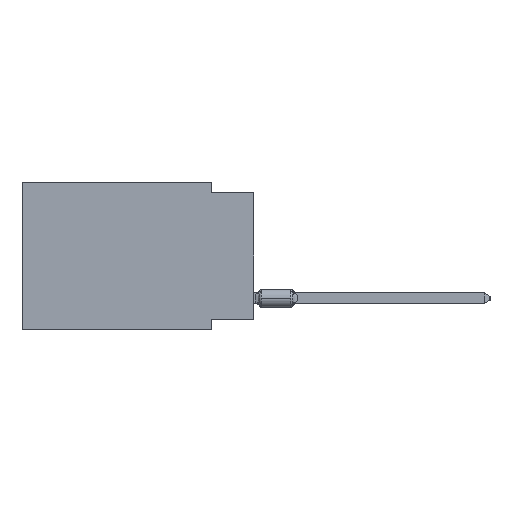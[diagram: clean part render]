
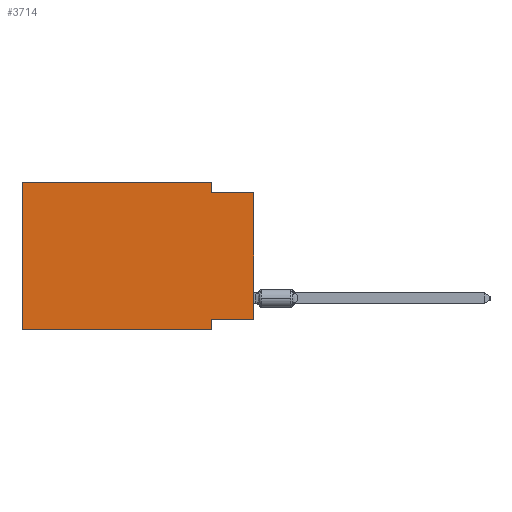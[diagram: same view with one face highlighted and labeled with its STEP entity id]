
A CAD part, left-side view. The second image highlights one B-rep face of the part: STEP entity #3714.
In plain terms, the highlighted planar face has unit normal (-1, 0, 0).
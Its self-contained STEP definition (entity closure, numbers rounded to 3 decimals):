
#231 = DIRECTION ( 'NONE',  ( 0., 0., 1. ) ) ;
#1166 = DIRECTION ( 'NONE',  ( 0., -1., 0. ) ) ;
#1847 = LINE ( 'NONE', #34086, #48528 ) ;
#1889 = EDGE_LOOP ( 'NONE', ( #29361, #66697, #50374, #24416, #51068, #53555, #51323, #31199 ) ) ;
#3714 = ADVANCED_FACE ( 'NONE', ( #41656 ), #31269, .F. ) ;
#4084 = EDGE_CURVE ( 'NONE', #60412, #12147, #8924, .T. ) ;
#4600 = DIRECTION ( 'NONE',  ( 0., -1., 0. ) ) ;
#6487 = EDGE_CURVE ( 'NONE', #22351, #21776, #40499, .T. ) ;
#8819 = EDGE_CURVE ( 'NONE', #22351, #29877, #49741, .T. ) ;
#8924 = LINE ( 'NONE', #9620, #40393 ) ;
#9620 = CARTESIAN_POINT ( 'NONE',  ( 0., 13.97, -8.89 ) ) ;
#9866 = VECTOR ( 'NONE', #20544, 1000. ) ;
#11893 = EDGE_CURVE ( 'NONE', #53885, #21776, #38814, .T. ) ;
#12147 = VERTEX_POINT ( 'NONE', #23573 ) ;
#13261 = VERTEX_POINT ( 'NONE', #54737 ) ;
#13292 = CARTESIAN_POINT ( 'NONE',  ( 0., 0., 0. ) ) ;
#13886 = CARTESIAN_POINT ( 'NONE',  ( 0., 0., -0.635 ) ) ;
#15494 = CARTESIAN_POINT ( 'NONE',  ( 0., 13.97, -8.89 ) ) ;
#16459 = DIRECTION ( 'NONE',  ( 0., 1., 0. ) ) ;
#19012 = DIRECTION ( 'NONE',  ( 0., 0., 1. ) ) ;
#20544 = DIRECTION ( 'NONE',  ( 0., 0., -1. ) ) ;
#21776 = VERTEX_POINT ( 'NONE', #13886 ) ;
#22351 = VERTEX_POINT ( 'NONE', #25579 ) ;
#22799 = LINE ( 'NONE', #48585, #66698 ) ;
#22912 = DIRECTION ( 'NONE',  ( 0., 0., -1. ) ) ;
#23573 = CARTESIAN_POINT ( 'NONE',  ( 0., 2.54, -8.89 ) ) ;
#24240 = VECTOR ( 'NONE', #19012, 1000. ) ;
#24416 = ORIENTED_EDGE ( 'NONE', *, *, #38826, .F. ) ;
#25579 = CARTESIAN_POINT ( 'NONE',  ( 0., 0., -8.255 ) ) ;
#25927 = LINE ( 'NONE', #63183, #9866 ) ;
#26893 = VECTOR ( 'NONE', #64623, 1000. ) ;
#27723 = CARTESIAN_POINT ( 'NONE',  ( 0., 0., -0.635 ) ) ;
#29361 = ORIENTED_EDGE ( 'NONE', *, *, #6487, .T. ) ;
#29877 = VERTEX_POINT ( 'NONE', #48621 ) ;
#31199 = ORIENTED_EDGE ( 'NONE', *, *, #8819, .F. ) ;
#31269 = PLANE ( 'NONE',  #43751 ) ;
#34086 = CARTESIAN_POINT ( 'NONE',  ( 0., 2.54, -8.89 ) ) ;
#35153 = DIRECTION ( 'NONE',  ( 0., 0., -1. ) ) ;
#38773 = LINE ( 'NONE', #60964, #41954 ) ;
#38814 = LINE ( 'NONE', #27723, #26893 ) ;
#38826 = EDGE_CURVE ( 'NONE', #13261, #70706, #38773, .T. ) ;
#39547 = EDGE_CURVE ( 'NONE', #60412, #13261, #22799, .T. ) ;
#40393 = VECTOR ( 'NONE', #4600, 1000. ) ;
#40499 = LINE ( 'NONE', #13292, #24240 ) ;
#41406 = CARTESIAN_POINT ( 'NONE',  ( 0., 2.54, 0. ) ) ;
#41656 = FACE_OUTER_BOUND ( 'NONE', #1889, .T. ) ;
#41954 = VECTOR ( 'NONE', #1166, 1000. ) ;
#42917 = CARTESIAN_POINT ( 'NONE',  ( 0., 2.54, -0.635 ) ) ;
#43751 = AXIS2_PLACEMENT_3D ( 'NONE', #53088, #63499, #22912 ) ;
#47110 = EDGE_CURVE ( 'NONE', #70706, #53885, #25927, .T. ) ;
#48528 = VECTOR ( 'NONE', #35153, 1000. ) ;
#48585 = CARTESIAN_POINT ( 'NONE',  ( 0., 13.97, 0. ) ) ;
#48621 = CARTESIAN_POINT ( 'NONE',  ( 0., 2.54, -8.255 ) ) ;
#49741 = LINE ( 'NONE', #66925, #60866 ) ;
#50374 = ORIENTED_EDGE ( 'NONE', *, *, #47110, .F. ) ;
#51068 = ORIENTED_EDGE ( 'NONE', *, *, #39547, .F. ) ;
#51323 = ORIENTED_EDGE ( 'NONE', *, *, #61839, .F. ) ;
#53088 = CARTESIAN_POINT ( 'NONE',  ( 0., 13.97, 0. ) ) ;
#53555 = ORIENTED_EDGE ( 'NONE', *, *, #4084, .T. ) ;
#53885 = VERTEX_POINT ( 'NONE', #42917 ) ;
#54737 = CARTESIAN_POINT ( 'NONE',  ( 0., 13.97, 0. ) ) ;
#60412 = VERTEX_POINT ( 'NONE', #15494 ) ;
#60866 = VECTOR ( 'NONE', #16459, 1000. ) ;
#60964 = CARTESIAN_POINT ( 'NONE',  ( 0., 13.97, 0. ) ) ;
#61839 = EDGE_CURVE ( 'NONE', #29877, #12147, #1847, .T. ) ;
#63183 = CARTESIAN_POINT ( 'NONE',  ( 0., 2.54, 0. ) ) ;
#63499 = DIRECTION ( 'NONE',  ( 1., 0., 0. ) ) ;
#64623 = DIRECTION ( 'NONE',  ( 0., -1., 0. ) ) ;
#66697 = ORIENTED_EDGE ( 'NONE', *, *, #11893, .F. ) ;
#66698 = VECTOR ( 'NONE', #231, 1000. ) ;
#66925 = CARTESIAN_POINT ( 'NONE',  ( 0., 0., -8.255 ) ) ;
#70706 = VERTEX_POINT ( 'NONE', #41406 ) ;
